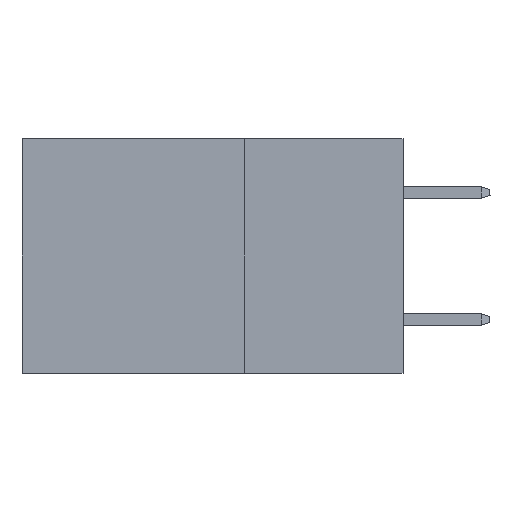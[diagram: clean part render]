
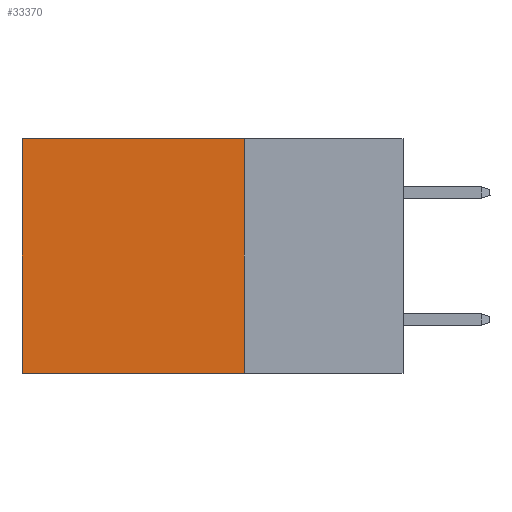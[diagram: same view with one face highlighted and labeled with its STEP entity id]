
A CAD part, left-side view. The second image highlights one B-rep face of the part: STEP entity #33370.
In plain terms, the highlighted planar face has unit normal (-1, 0, 0).
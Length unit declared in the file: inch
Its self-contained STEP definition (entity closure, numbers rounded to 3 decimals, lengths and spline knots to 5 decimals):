
#226 = EDGE_CURVE ( 'NONE', #14694, #10681, #22033, .T. ) ;
#753 = ORIENTED_EDGE ( 'NONE', *, *, #24226, .T. ) ;
#5991 = VERTEX_POINT ( 'NONE', #29597 ) ;
#6710 = DIRECTION ( 'NONE',  ( 0., 0., -1. ) ) ;
#7264 = DIRECTION ( 'NONE',  ( 0., 1., 0. ) ) ;
#8742 = VECTOR ( 'NONE', #34781, 39.37008 ) ;
#8821 = VECTOR ( 'NONE', #6710, 39.37008 ) ;
#8834 = DIRECTION ( 'NONE',  ( 1., 0., 0. ) ) ;
#9358 = LINE ( 'NONE', #20725, #8821 ) ;
#10500 = EDGE_LOOP ( 'NONE', ( #753, #28379, #24715, #26033 ) ) ;
#10681 = VERTEX_POINT ( 'NONE', #18848 ) ;
#12727 = CARTESIAN_POINT ( 'NONE',  ( 0.2875, 0.25, -0.37 ) ) ;
#13968 = VECTOR ( 'NONE', #7264, 39.37008 ) ;
#14057 = FACE_OUTER_BOUND ( 'NONE', #10500, .T. ) ;
#14694 = VERTEX_POINT ( 'NONE', #12727 ) ;
#14962 = LINE ( 'NONE', #25983, #8742 ) ;
#15859 = CARTESIAN_POINT ( 'NONE',  ( 0.2875, 0.25, -0.37 ) ) ;
#16266 = EDGE_CURVE ( 'NONE', #34148, #5991, #14962, .T. ) ;
#17230 = PLANE ( 'NONE',  #20389 ) ;
#17397 = EDGE_CURVE ( 'NONE', #34148, #14694, #9358, .T. ) ;
#18848 = CARTESIAN_POINT ( 'NONE',  ( 0.2875, 0.6, -0.37 ) ) ;
#20157 = LINE ( 'NONE', #25611, #32044 ) ;
#20389 = AXIS2_PLACEMENT_3D ( 'NONE', #22678, #8834, #25470 ) ;
#20725 = CARTESIAN_POINT ( 'NONE',  ( 0.2875, 0.25, 0. ) ) ;
#22033 = LINE ( 'NONE', #15859, #13968 ) ;
#22678 = CARTESIAN_POINT ( 'NONE',  ( 0.2875, 0.25, 0. ) ) ;
#24226 = EDGE_CURVE ( 'NONE', #5991, #10681, #20157, .T. ) ;
#24715 = ORIENTED_EDGE ( 'NONE', *, *, #17397, .F. ) ;
#25000 = CARTESIAN_POINT ( 'NONE',  ( 0.2875, 0.25, 0. ) ) ;
#25470 = DIRECTION ( 'NONE',  ( 0., 0., -1. ) ) ;
#25611 = CARTESIAN_POINT ( 'NONE',  ( 0.2875, 0.6, 0. ) ) ;
#25983 = CARTESIAN_POINT ( 'NONE',  ( 0.2875, 0.25, 0. ) ) ;
#26033 = ORIENTED_EDGE ( 'NONE', *, *, #16266, .T. ) ;
#28379 = ORIENTED_EDGE ( 'NONE', *, *, #226, .F. ) ;
#29597 = CARTESIAN_POINT ( 'NONE',  ( 0.2875, 0.6, 0. ) ) ;
#31567 = DIRECTION ( 'NONE',  ( 0., 0., -1. ) ) ;
#32044 = VECTOR ( 'NONE', #31567, 39.37008 ) ;
#33370 = ADVANCED_FACE ( 'NONE', ( #14057 ), #17230, .F. ) ;
#34148 = VERTEX_POINT ( 'NONE', #25000 ) ;
#34781 = DIRECTION ( 'NONE',  ( 0., 1., 0. ) ) ;
